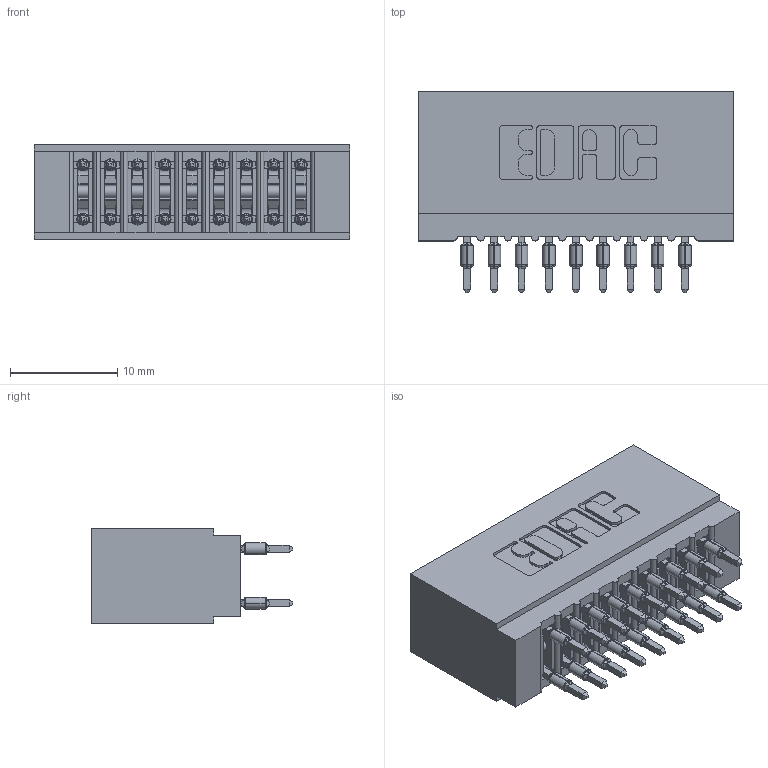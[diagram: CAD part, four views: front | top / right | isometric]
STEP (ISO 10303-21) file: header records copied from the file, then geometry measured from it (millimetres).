
FILE_DESCRIPTION (( 'STEP AP203' ), '1' );
FILE_NAME ('725-018-560-201.STEP', '2026-02-24T16:48:30', ( '' ), ( '' ), 'SwSTEP 2.0', 'SolidWorks 2023', '' );
FILE_SCHEMA (( 'CONFIG_CONTROL_DESIGN' ));
Length unit declared in the file: millimetre
Products named in the file (3): 745-292-001_560; 725 Part_Insulator Option - 01; 725-018-560-201
Assembly tree (19 placements, depth 2):
  725-018-560-201
    725 Part_Insulator Option - 01
    745-292-001_560  x18
Bounding box: 29.46 x 18.8 x 8.89 mm (x, y, z)
Volume: 2569.3 mm3; surface area: 5004.7 mm2
Topology: 19 solids, 19 shells, 1868 faces, 5105 edges, 3246 vertices
Faces by surface type: plane 973, cylinder 427, bspline 360, torus 108
Entity records: 19944 total; most frequent: CARTESIAN_POINT 3973, ORIENTED_EDGE 3342, DIRECTION 2955, EDGE_CURVE 1671, VECTOR 1427, LINE 1427, VERTEX_POINT 1070, AXIS2_PLACEMENT_3D 764
